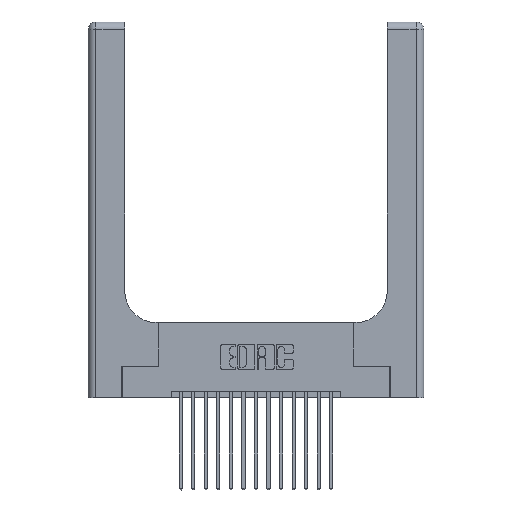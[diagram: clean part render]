
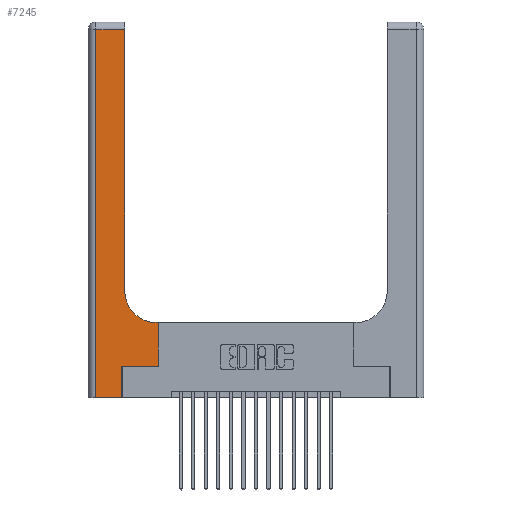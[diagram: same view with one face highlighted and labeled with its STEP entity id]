
A CAD part, top view. The second image highlights one B-rep face of the part: STEP entity #7245.
In plain terms, the highlighted planar face has unit normal (0, 0, 1).
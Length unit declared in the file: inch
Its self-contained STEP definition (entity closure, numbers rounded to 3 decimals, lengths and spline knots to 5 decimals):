
#81 = LINE ( 'NONE', #8485, #18507 ) ;
#90 = DIRECTION ( 'NONE',  ( -1., 0., 0. ) ) ;
#451 = VERTEX_POINT ( 'NONE', #15535 ) ;
#536 = DIRECTION ( 'NONE',  ( 1., 0., 0. ) ) ;
#672 = EDGE_CURVE ( 'NONE', #3928, #16588, #851, .T. ) ;
#816 = LINE ( 'NONE', #10936, #9914 ) ;
#851 = LINE ( 'NONE', #8230, #9039 ) ;
#1039 = EDGE_CURVE ( 'NONE', #16588, #451, #12739, .T. ) ;
#1568 = EDGE_CURVE ( 'NONE', #17634, #4149, #5521, .T. ) ;
#3208 = CARTESIAN_POINT ( 'NONE',  ( 0.5415, 0.85, 0.37 ) ) ;
#3380 = LINE ( 'NONE', #4705, #17126 ) ;
#3570 = EDGE_CURVE ( 'NONE', #17291, #9752, #81, .T. ) ;
#3928 = VERTEX_POINT ( 'NONE', #19241 ) ;
#4149 = VERTEX_POINT ( 'NONE', #13155 ) ;
#4698 = DIRECTION ( 'NONE',  ( 0., 0., -1. ) ) ;
#4705 = CARTESIAN_POINT ( 'NONE',  ( 0.269, 0., 0.37 ) ) ;
#4970 = DIRECTION ( 'NONE',  ( 0., 0., -1. ) ) ;
#5521 = LINE ( 'NONE', #6303, #14845 ) ;
#5565 = EDGE_CURVE ( 'NONE', #12698, #17291, #12372, .T. ) ;
#5799 = CARTESIAN_POINT ( 'NONE',  ( 0.06, 2.94, 0.37 ) ) ;
#6303 = CARTESIAN_POINT ( 'NONE',  ( 0.269, 0.25, 0.37 ) ) ;
#6322 = VECTOR ( 'NONE', #18463, 39.37008 ) ;
#6341 = ORIENTED_EDGE ( 'NONE', *, *, #3570, .T. ) ;
#6735 = CARTESIAN_POINT ( 'NONE',  ( 0.2915, 2.94, 0.37 ) ) ;
#6888 = AXIS2_PLACEMENT_3D ( 'NONE', #13669, #4698, #90 ) ;
#7245 = ADVANCED_FACE ( 'NONE', ( #12123 ), #16643, .F. ) ;
#7699 = DIRECTION ( 'NONE',  ( 1., 0., 0. ) ) ;
#7792 = ORIENTED_EDGE ( 'NONE', *, *, #15536, .T. ) ;
#7891 = DIRECTION ( 'NONE',  ( 0., 1., 0. ) ) ;
#8052 = CARTESIAN_POINT ( 'NONE',  ( 0.06, 3., 0.37 ) ) ;
#8163 = DIRECTION ( 'NONE',  ( -1., 0., 0. ) ) ;
#8230 = CARTESIAN_POINT ( 'NONE',  ( 0.2915, 0.6, 0.37 ) ) ;
#8354 = DIRECTION ( 'NONE',  ( 1., 0., 0. ) ) ;
#8485 = CARTESIAN_POINT ( 'NONE',  ( 0., 0., 0.37 ) ) ;
#9005 = CARTESIAN_POINT ( 'NONE',  ( 0.06, 0., 0.37 ) ) ;
#9039 = VECTOR ( 'NONE', #8163, 39.37008 ) ;
#9574 = CARTESIAN_POINT ( 'NONE',  ( 0.269, 0.25, 0.37 ) ) ;
#9752 = VERTEX_POINT ( 'NONE', #11474 ) ;
#9914 = VECTOR ( 'NONE', #7891, 39.37008 ) ;
#10153 = VERTEX_POINT ( 'NONE', #6735 ) ;
#10349 = VECTOR ( 'NONE', #17025, 39.37008 ) ;
#10936 = CARTESIAN_POINT ( 'NONE',  ( 0.5585, 0.25, 0.37 ) ) ;
#11471 = ORIENTED_EDGE ( 'NONE', *, *, #672, .T. ) ;
#11474 = CARTESIAN_POINT ( 'NONE',  ( 0.269, 0., 0.37 ) ) ;
#11722 = EDGE_CURVE ( 'NONE', #451, #10153, #16596, .T. ) ;
#11859 = ORIENTED_EDGE ( 'NONE', *, *, #5565, .T. ) ;
#12123 = FACE_OUTER_BOUND ( 'NONE', #15609, .T. ) ;
#12372 = LINE ( 'NONE', #8052, #6322 ) ;
#12459 = ORIENTED_EDGE ( 'NONE', *, *, #15943, .T. ) ;
#12698 = VERTEX_POINT ( 'NONE', #5799 ) ;
#12739 = CIRCLE ( 'NONE', #19004, 0.25 ) ;
#13155 = CARTESIAN_POINT ( 'NONE',  ( 0.5585, 0.25, 0.37 ) ) ;
#13391 = LINE ( 'NONE', #17155, #10349 ) ;
#13669 = CARTESIAN_POINT ( 'NONE',  ( 0., 3., 0.37 ) ) ;
#14845 = VECTOR ( 'NONE', #536, 39.37008 ) ;
#15117 = DIRECTION ( 'NONE',  ( 0., 1., 0. ) ) ;
#15198 = DIRECTION ( 'NONE',  ( 0., 1., 0. ) ) ;
#15535 = CARTESIAN_POINT ( 'NONE',  ( 0.2915, 0.85, 0.37 ) ) ;
#15536 = EDGE_CURVE ( 'NONE', #4149, #3928, #816, .T. ) ;
#15609 = EDGE_LOOP ( 'NONE', ( #18969, #15958, #11859, #6341, #12459, #19059, #7792, #11471, #18323 ) ) ;
#15943 = EDGE_CURVE ( 'NONE', #9752, #17634, #3380, .T. ) ;
#15958 = ORIENTED_EDGE ( 'NONE', *, *, #18096, .T. ) ;
#16375 = CARTESIAN_POINT ( 'NONE',  ( 0.5415, 0.6, 0.37 ) ) ;
#16588 = VERTEX_POINT ( 'NONE', #16375 ) ;
#16596 = LINE ( 'NONE', #18161, #19174 ) ;
#16643 = PLANE ( 'NONE',  #6888 ) ;
#17025 = DIRECTION ( 'NONE',  ( -1., 0., 0. ) ) ;
#17126 = VECTOR ( 'NONE', #15117, 39.37008 ) ;
#17155 = CARTESIAN_POINT ( 'NONE',  ( 0., 2.94, 0.37 ) ) ;
#17291 = VERTEX_POINT ( 'NONE', #9005 ) ;
#17634 = VERTEX_POINT ( 'NONE', #9574 ) ;
#18096 = EDGE_CURVE ( 'NONE', #10153, #12698, #13391, .T. ) ;
#18161 = CARTESIAN_POINT ( 'NONE',  ( 0.2915, 3., 0.37 ) ) ;
#18323 = ORIENTED_EDGE ( 'NONE', *, *, #1039, .T. ) ;
#18463 = DIRECTION ( 'NONE',  ( 0., -1., 0. ) ) ;
#18507 = VECTOR ( 'NONE', #8354, 39.37008 ) ;
#18969 = ORIENTED_EDGE ( 'NONE', *, *, #11722, .T. ) ;
#19004 = AXIS2_PLACEMENT_3D ( 'NONE', #3208, #4970, #7699 ) ;
#19059 = ORIENTED_EDGE ( 'NONE', *, *, #1568, .T. ) ;
#19174 = VECTOR ( 'NONE', #15198, 39.37008 ) ;
#19241 = CARTESIAN_POINT ( 'NONE',  ( 0.5585, 0.6, 0.37 ) ) ;
